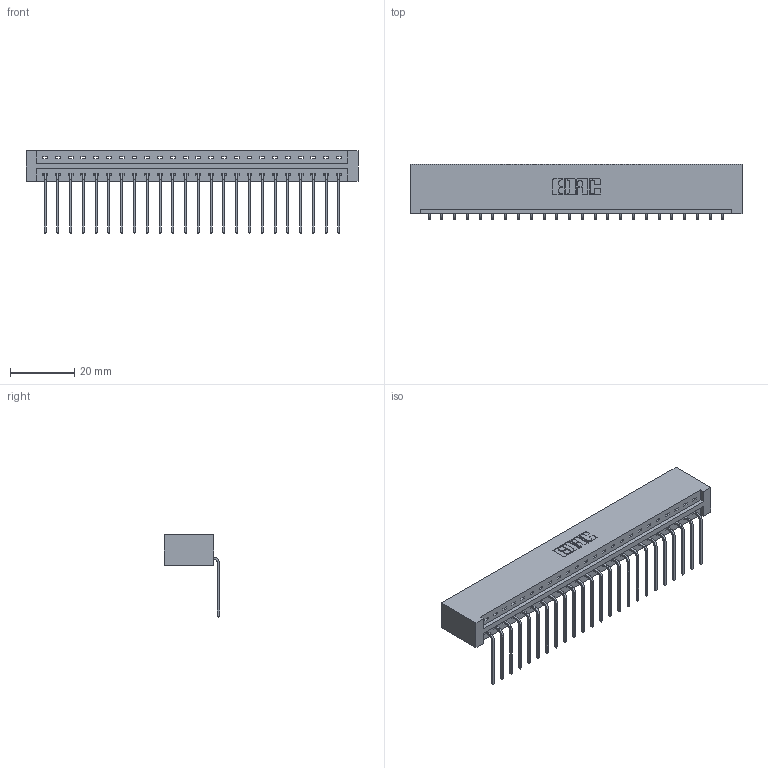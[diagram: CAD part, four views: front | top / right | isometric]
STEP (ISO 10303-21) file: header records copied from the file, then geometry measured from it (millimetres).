
FILE_DESCRIPTION (( 'STEP AP203' ), '1' );
FILE_NAME ('337-024-559-101.STEP', '2019-09-30T16:11:22', ( '' ), ( '' ), 'SwSTEP 2.0', 'SolidWorks 2016', '' );
FILE_SCHEMA (( 'CONFIG_CONTROL_DESIGN' ));
Length unit declared in the file: inch
Products named in the file (3): 337 Part_No Mounting Lugs; 337-024-559-101; 345-292-001_558 559 Tail - 1
Assembly tree (25 placements, depth 2):
  337-024-559-101
    337 Part_No Mounting Lugs
    345-292-001_558 559 Tail - 1  x24
Bounding box: 102.97 x 17.09 x 25.53 mm (x, y, z)
Volume: 11295.6 mm3; surface area: 12045.1 mm2
Topology: 25 solids, 25 shells, 1642 faces, 4943 edges, 3262 vertices
Faces by surface type: plane 1218, cylinder 424
Entity records: 19975 total; most frequent: CARTESIAN_POINT 3486, ORIENTED_EDGE 3446, DIRECTION 2963, EDGE_CURVE 1723, LINE 1603, VECTOR 1603, VERTEX_POINT 1146, AXIS2_PLACEMENT_3D 680
